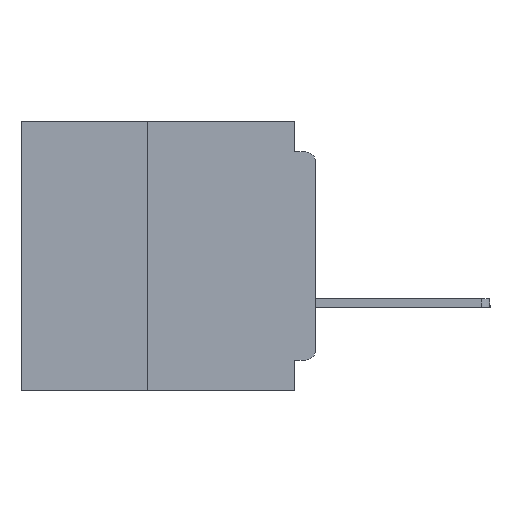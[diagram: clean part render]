
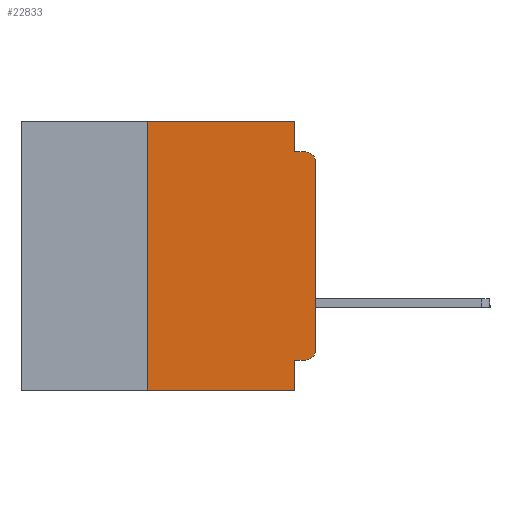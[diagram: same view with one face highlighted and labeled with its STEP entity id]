
A CAD part, left-side view. The second image highlights one B-rep face of the part: STEP entity #22833.
In plain terms, the highlighted planar face has unit normal (-1, 0, 0).
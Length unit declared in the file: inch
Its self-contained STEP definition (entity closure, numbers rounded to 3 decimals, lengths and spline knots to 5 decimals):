
#100 = DIRECTION ( 'NONE',  ( 0., -1., 0. ) ) ;
#758 = CARTESIAN_POINT ( 'NONE',  ( 0., 0., 0. ) ) ;
#2457 = CARTESIAN_POINT ( 'NONE',  ( 0., 0.25, 0. ) ) ;
#2740 = CARTESIAN_POINT ( 'NONE',  ( 0., 0.437, 0. ) ) ;
#2808 = VERTEX_POINT ( 'NONE', #2878 ) ;
#2878 = CARTESIAN_POINT ( 'NONE',  ( 0., 0.031, -0.045 ) ) ;
#3811 = CARTESIAN_POINT ( 'NONE',  ( 0., 0.031, -0.4 ) ) ;
#5377 = VERTEX_POINT ( 'NONE', #2457 ) ;
#5934 = EDGE_CURVE ( 'NONE', #30590, #5377, #7539, .T. ) ;
#6172 = VERTEX_POINT ( 'NONE', #43723 ) ;
#6936 = DIRECTION ( 'NONE',  ( -1., 0., 0. ) ) ;
#7443 = DIRECTION ( 'NONE',  ( 0., 1., 0. ) ) ;
#7539 = LINE ( 'NONE', #47852, #20742 ) ;
#8242 = DIRECTION ( 'NONE',  ( 0., 0., 1. ) ) ;
#8763 = DIRECTION ( 'NONE',  ( 0., 0., -1. ) ) ;
#8850 = CARTESIAN_POINT ( 'NONE',  ( 0., 0., -0.06 ) ) ;
#9493 = CARTESIAN_POINT ( 'NONE',  ( 0., 0.015, -0.045 ) ) ;
#9721 = EDGE_CURVE ( 'NONE', #5377, #6172, #39471, .T. ) ;
#10735 = ORIENTED_EDGE ( 'NONE', *, *, #40070, .T. ) ;
#11513 = LINE ( 'NONE', #13164, #47866 ) ;
#11580 = ORIENTED_EDGE ( 'NONE', *, *, #39546, .T. ) ;
#12098 = ORIENTED_EDGE ( 'NONE', *, *, #22893, .F. ) ;
#12450 = CARTESIAN_POINT ( 'NONE',  ( 0., 0.437, -0.4 ) ) ;
#12748 = PLANE ( 'NONE',  #31772 ) ;
#12878 = EDGE_CURVE ( 'NONE', #13997, #37494, #33339, .T. ) ;
#13078 = FACE_OUTER_BOUND ( 'NONE', #44790, .T. ) ;
#13164 = CARTESIAN_POINT ( 'NONE',  ( 0., 0., -0.045 ) ) ;
#13997 = VERTEX_POINT ( 'NONE', #59763 ) ;
#14002 = ORIENTED_EDGE ( 'NONE', *, *, #20775, .F. ) ;
#14185 = ORIENTED_EDGE ( 'NONE', *, *, #9721, .F. ) ;
#16851 = ORIENTED_EDGE ( 'NONE', *, *, #5934, .F. ) ;
#16905 = ORIENTED_EDGE ( 'NONE', *, *, #37223, .T. ) ;
#17735 = DIRECTION ( 'NONE',  ( 0., 0., -1. ) ) ;
#18007 = CARTESIAN_POINT ( 'NONE',  ( 0., 0., -0.34 ) ) ;
#18171 = DIRECTION ( 'NONE',  ( 0., -1., 0. ) ) ;
#18680 = VECTOR ( 'NONE', #7443, 39.37008 ) ;
#18856 = ORIENTED_EDGE ( 'NONE', *, *, #12878, .F. ) ;
#19000 = ORIENTED_EDGE ( 'NONE', *, *, #52327, .F. ) ;
#19118 = ORIENTED_EDGE ( 'NONE', *, *, #51079, .T. ) ;
#19559 = VERTEX_POINT ( 'NONE', #9493 ) ;
#20333 = VERTEX_POINT ( 'NONE', #8850 ) ;
#20742 = VECTOR ( 'NONE', #8242, 39.37008 ) ;
#20775 = EDGE_CURVE ( 'NONE', #6172, #2808, #61415, .T. ) ;
#22833 = ADVANCED_FACE ( 'NONE', ( #13078 ), #12748, .F. ) ;
#22893 = EDGE_CURVE ( 'NONE', #2808, #19559, #11513, .T. ) ;
#24892 = VECTOR ( 'NONE', #100, 39.37008 ) ;
#26476 = CARTESIAN_POINT ( 'NONE',  ( 0., 0.015, -0.34 ) ) ;
#27524 = VERTEX_POINT ( 'NONE', #42838 ) ;
#28431 = CARTESIAN_POINT ( 'NONE',  ( 0., 0.25, -0.4 ) ) ;
#29874 = CARTESIAN_POINT ( 'NONE',  ( 0., 0.437, 0. ) ) ;
#30590 = VERTEX_POINT ( 'NONE', #28431 ) ;
#31479 = DIRECTION ( 'NONE',  ( 0., 0., -1. ) ) ;
#31772 = AXIS2_PLACEMENT_3D ( 'NONE', #2740, #47317, #17735 ) ;
#31827 = VECTOR ( 'NONE', #8763, 39.37008 ) ;
#32056 = CARTESIAN_POINT ( 'NONE',  ( 0., 0.031, 0. ) ) ;
#32195 = CARTESIAN_POINT ( 'NONE',  ( 0., 0., -0.355 ) ) ;
#33339 = LINE ( 'NONE', #3811, #31827 ) ;
#33701 = VECTOR ( 'NONE', #51895, 39.37008 ) ;
#33994 = LINE ( 'NONE', #12450, #60172 ) ;
#36573 = CARTESIAN_POINT ( 'NONE',  ( 0., 0.015, -0.06 ) ) ;
#37223 = EDGE_CURVE ( 'NONE', #30590, #37494, #33994, .T. ) ;
#37494 = VERTEX_POINT ( 'NONE', #48926 ) ;
#39471 = LINE ( 'NONE', #29874, #24892 ) ;
#39546 = EDGE_CURVE ( 'NONE', #20333, #19559, #61485, .T. ) ;
#40070 = EDGE_CURVE ( 'NONE', #53865, #20333, #60489, .T. ) ;
#40509 = AXIS2_PLACEMENT_3D ( 'NONE', #36573, #6936, #41535 ) ;
#41535 = DIRECTION ( 'NONE',  ( 0., 0., -1. ) ) ;
#42838 = CARTESIAN_POINT ( 'NONE',  ( 0., 0.015, -0.355 ) ) ;
#43723 = CARTESIAN_POINT ( 'NONE',  ( 0., 0.031, 0. ) ) ;
#44019 = CIRCLE ( 'NONE', #58767, 0.015 ) ;
#44790 = EDGE_LOOP ( 'NONE', ( #10735, #11580, #12098, #14002, #14185, #16851, #16905, #18856, #19000, #19118 ) ) ;
#46519 = LINE ( 'NONE', #32195, #18680 ) ;
#47317 = DIRECTION ( 'NONE',  ( 1., 0., 0. ) ) ;
#47447 = VECTOR ( 'NONE', #60185, 39.37008 ) ;
#47852 = CARTESIAN_POINT ( 'NONE',  ( 0., 0.25, -0.4 ) ) ;
#47866 = VECTOR ( 'NONE', #18171, 39.37008 ) ;
#48926 = CARTESIAN_POINT ( 'NONE',  ( 0., 0.031, -0.4 ) ) ;
#51079 = EDGE_CURVE ( 'NONE', #27524, #53865, #44019, .T. ) ;
#51895 = DIRECTION ( 'NONE',  ( 0., 0., -1. ) ) ;
#52327 = EDGE_CURVE ( 'NONE', #27524, #13997, #46519, .T. ) ;
#53865 = VERTEX_POINT ( 'NONE', #18007 ) ;
#58767 = AXIS2_PLACEMENT_3D ( 'NONE', #26476, #60903, #31479 ) ;
#59763 = CARTESIAN_POINT ( 'NONE',  ( 0., 0.031, -0.355 ) ) ;
#60172 = VECTOR ( 'NONE', #61609, 39.37008 ) ;
#60185 = DIRECTION ( 'NONE',  ( 0., 0., 1. ) ) ;
#60489 = LINE ( 'NONE', #758, #47447 ) ;
#60903 = DIRECTION ( 'NONE',  ( -1., 0., 0. ) ) ;
#61415 = LINE ( 'NONE', #32056, #33701 ) ;
#61485 = CIRCLE ( 'NONE', #40509, 0.015 ) ;
#61609 = DIRECTION ( 'NONE',  ( 0., -1., 0. ) ) ;
